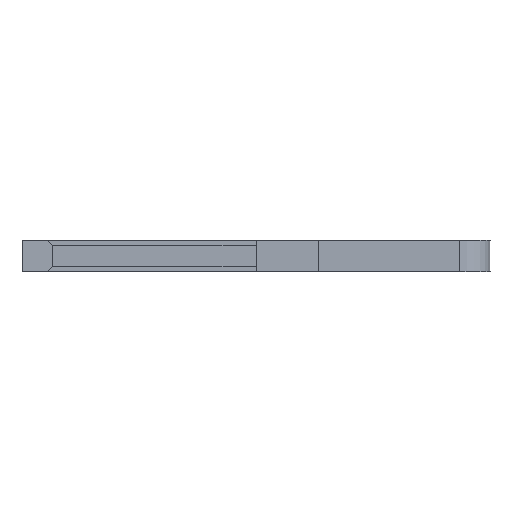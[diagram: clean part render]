
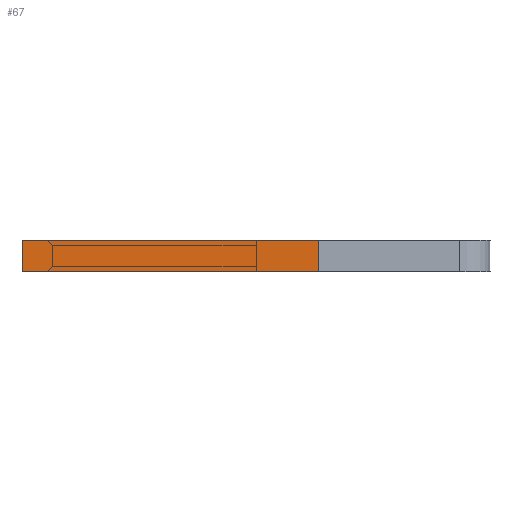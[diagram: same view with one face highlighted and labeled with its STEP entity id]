
A CAD part, left-side view. The second image highlights one B-rep face of the part: STEP entity #67.
In plain terms, the highlighted face is planar.
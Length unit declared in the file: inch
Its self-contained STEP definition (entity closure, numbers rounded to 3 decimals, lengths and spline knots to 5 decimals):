
#22 = ORIENTED_EDGE ( 'NONE', *, *, #498, .F. ) ;
#67 = ADVANCED_FACE ( 'NONE', ( #806 ), #2279, .F. ) ;
#137 = CARTESIAN_POINT ( 'NONE',  ( -0.01, -0.04, -0.04 ) ) ;
#222 = EDGE_CURVE ( 'NONE', #1673, #381, #739, .T. ) ;
#381 = VERTEX_POINT ( 'NONE', #2091 ) ;
#413 = DIRECTION ( 'NONE',  ( 0., 1., 0. ) ) ;
#418 = ORIENTED_EDGE ( 'NONE', *, *, #222, .T. ) ;
#438 = LINE ( 'NONE', #1609, #2068 ) ;
#498 = EDGE_CURVE ( 'NONE', #2560, #2704, #2076, .T. ) ;
#739 = LINE ( 'NONE', #1663, #1089 ) ;
#805 = EDGE_LOOP ( 'NONE', ( #418, #938, #22, #2080 ) ) ;
#806 = FACE_OUTER_BOUND ( 'NONE', #805, .T. ) ;
#861 = DIRECTION ( 'NONE',  ( -1., 0., 0. ) ) ;
#938 = ORIENTED_EDGE ( 'NONE', *, *, #941, .F. ) ;
#939 = VECTOR ( 'NONE', #413, 39.37008 ) ;
#941 = EDGE_CURVE ( 'NONE', #2704, #381, #1532, .T. ) ;
#1089 = VECTOR ( 'NONE', #2329, 39.37008 ) ;
#1119 = VECTOR ( 'NONE', #861, 39.37008 ) ;
#1212 = DIRECTION ( 'NONE',  ( 1., 0., 0. ) ) ;
#1222 = CARTESIAN_POINT ( 'NONE',  ( 0.01, 0.15, -0.04 ) ) ;
#1249 = CARTESIAN_POINT ( 'NONE',  ( 0.01, 0.15, -0.04 ) ) ;
#1366 = DIRECTION ( 'NONE',  ( -1., 0., 0. ) ) ;
#1454 = DIRECTION ( 'NONE',  ( 0., 0., 1. ) ) ;
#1465 = CARTESIAN_POINT ( 'NONE',  ( 0.01, 0.15, -0.04 ) ) ;
#1469 = AXIS2_PLACEMENT_3D ( 'NONE', #1249, #1454, #1212 ) ;
#1532 = LINE ( 'NONE', #2352, #1119 ) ;
#1609 = CARTESIAN_POINT ( 'NONE',  ( 0.01, -0.04, -0.04 ) ) ;
#1663 = CARTESIAN_POINT ( 'NONE',  ( -0.01, 0.15, -0.04 ) ) ;
#1673 = VERTEX_POINT ( 'NONE', #137 ) ;
#1692 = CARTESIAN_POINT ( 'NONE',  ( 0.01, -0.04, -0.04 ) ) ;
#2068 = VECTOR ( 'NONE', #1366, 39.37008 ) ;
#2076 = LINE ( 'NONE', #1222, #939 ) ;
#2080 = ORIENTED_EDGE ( 'NONE', *, *, #2130, .T. ) ;
#2091 = CARTESIAN_POINT ( 'NONE',  ( -0.01, 0.15, -0.04 ) ) ;
#2130 = EDGE_CURVE ( 'NONE', #2560, #1673, #438, .T. ) ;
#2279 = PLANE ( 'NONE',  #1469 ) ;
#2329 = DIRECTION ( 'NONE',  ( 0., 1., 0. ) ) ;
#2352 = CARTESIAN_POINT ( 'NONE',  ( 0.01, 0.15, -0.04 ) ) ;
#2560 = VERTEX_POINT ( 'NONE', #1692 ) ;
#2704 = VERTEX_POINT ( 'NONE', #1465 ) ;
